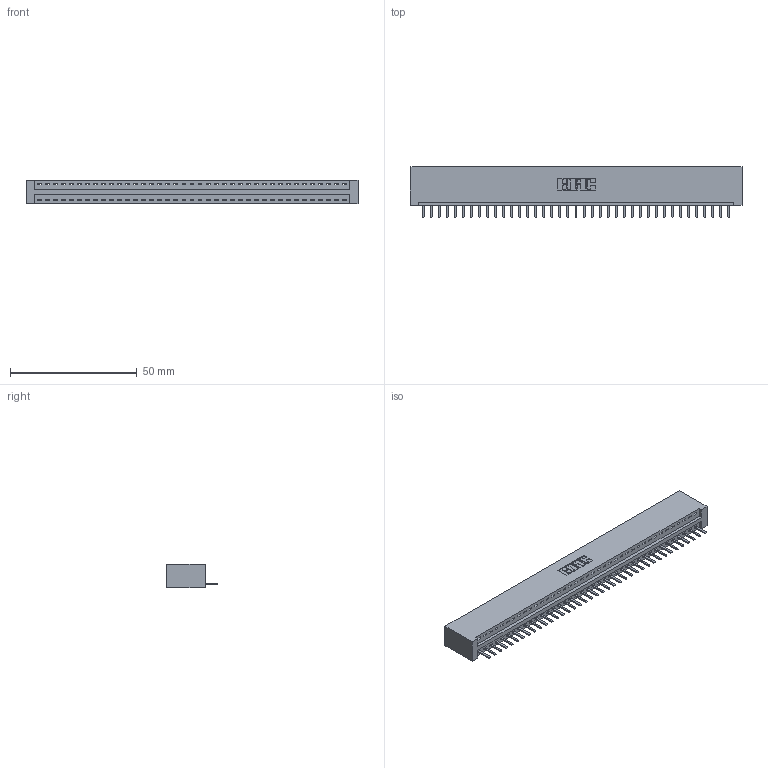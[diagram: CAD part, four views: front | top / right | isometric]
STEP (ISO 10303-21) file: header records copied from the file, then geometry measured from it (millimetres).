
FILE_DESCRIPTION (( 'STEP AP203' ), '1' );
FILE_NAME ('396-039-520-101.STEP', '2019-10-27T18:50:31', ( '' ), ( '' ), 'SwSTEP 2.0', 'SolidWorks 2016', '' );
FILE_SCHEMA (( 'CONFIG_CONTROL_DESIGN' ));
Length unit declared in the file: inch
Products named in the file (3): 396-039-520-101; 345-292-001_345-293-120; 346 Part_No Mounting Lugs
Assembly tree (40 placements, depth 2):
  396-039-520-101
    346 Part_No Mounting Lugs
    345-292-001_345-293-120  x39
Bounding box: 131.06 x 20.02 x 9.4 mm (x, y, z)
Volume: 12962.3 mm3; surface area: 15869.4 mm2
Topology: 40 solids, 40 shells, 2532 faces, 7481 edges, 4882 vertices
Faces by surface type: plane 1710, cylinder 822
Entity records: 24445 total; most frequent: CARTESIAN_POINT 4209, ORIENTED_EDGE 4170, DIRECTION 3699, EDGE_CURVE 2085, LINE 1801, VECTOR 1801, VERTEX_POINT 1386, AXIS2_PLACEMENT_3D 949
